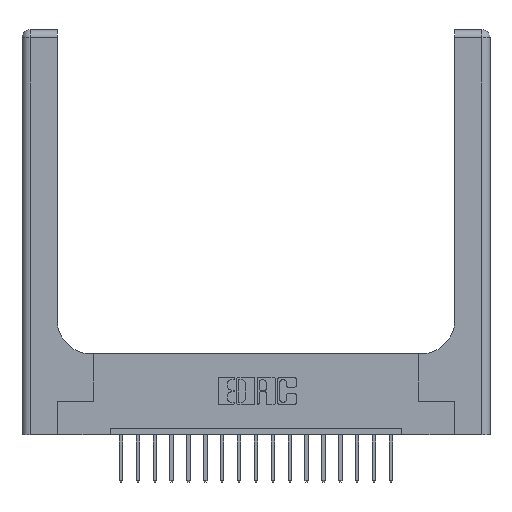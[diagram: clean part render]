
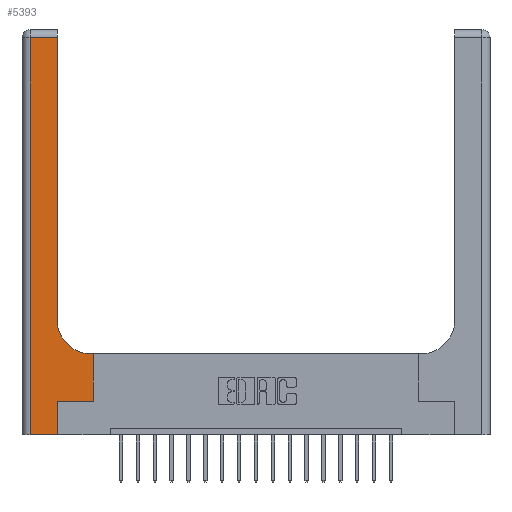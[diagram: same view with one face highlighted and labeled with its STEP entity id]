
A CAD part, top view. The second image highlights one B-rep face of the part: STEP entity #5393.
In plain terms, the highlighted planar face has unit normal (0, 0, 1).
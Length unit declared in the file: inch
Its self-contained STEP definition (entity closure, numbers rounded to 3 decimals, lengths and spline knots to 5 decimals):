
#104 = DIRECTION ( 'NONE',  ( 0., 0., -1. ) ) ;
#293 = FACE_OUTER_BOUND ( 'NONE', #8924, .T. ) ;
#439 = DIRECTION ( 'NONE',  ( 0., 1., 0. ) ) ;
#589 = CARTESIAN_POINT ( 'NONE',  ( 0.26, 0.6, 0.37 ) ) ;
#680 = DIRECTION ( 'NONE',  ( 1., 0., 0. ) ) ;
#683 = ORIENTED_EDGE ( 'NONE', *, *, #4215, .T. ) ;
#714 = DIRECTION ( 'NONE',  ( -1., 0., 0. ) ) ;
#737 = CARTESIAN_POINT ( 'NONE',  ( 0.528, 0.25, 0.37 ) ) ;
#1125 = EDGE_CURVE ( 'NONE', #5862, #8726, #2071, .T. ) ;
#1465 = CARTESIAN_POINT ( 'NONE',  ( 0.528, 0.6, 0.37 ) ) ;
#2071 = LINE ( 'NONE', #589, #18342 ) ;
#2080 = VERTEX_POINT ( 'NONE', #737 ) ;
#2270 = DIRECTION ( 'NONE',  ( -1., 0., 0. ) ) ;
#2566 = CARTESIAN_POINT ( 'NONE',  ( 0.265, 0., 0.37 ) ) ;
#2879 = VERTEX_POINT ( 'NONE', #10970 ) ;
#2986 = ORIENTED_EDGE ( 'NONE', *, *, #13654, .T. ) ;
#3689 = LINE ( 'NONE', #17036, #10026 ) ;
#4020 = DIRECTION ( 'NONE',  ( 1., 0., 0. ) ) ;
#4074 = AXIS2_PLACEMENT_3D ( 'NONE', #7520, #8815, #10492 ) ;
#4215 = EDGE_CURVE ( 'NONE', #8726, #6994, #14821, .T. ) ;
#4394 = VERTEX_POINT ( 'NONE', #2566 ) ;
#4497 = DIRECTION ( 'NONE',  ( 0., 1., 0. ) ) ;
#4581 = VECTOR ( 'NONE', #4020, 39.37008 ) ;
#5181 = CARTESIAN_POINT ( 'NONE',  ( 0.26, 3., 0.37 ) ) ;
#5393 = ADVANCED_FACE ( 'NONE', ( #293 ), #18110, .F. ) ;
#5862 = VERTEX_POINT ( 'NONE', #1465 ) ;
#6149 = DIRECTION ( 'NONE',  ( -1., 0., 0. ) ) ;
#6428 = EDGE_CURVE ( 'NONE', #4394, #15464, #8164, .T. ) ;
#6541 = ORIENTED_EDGE ( 'NONE', *, *, #6428, .T. ) ;
#6583 = CARTESIAN_POINT ( 'NONE',  ( 0.265, 0., 0.37 ) ) ;
#6991 = LINE ( 'NONE', #11636, #4581 ) ;
#6994 = VERTEX_POINT ( 'NONE', #19374 ) ;
#7324 = ORIENTED_EDGE ( 'NONE', *, *, #13899, .T. ) ;
#7430 = LINE ( 'NONE', #13553, #15594 ) ;
#7520 = CARTESIAN_POINT ( 'NONE',  ( 0.51, 0.85, 0.37 ) ) ;
#7566 = CARTESIAN_POINT ( 'NONE',  ( 0.528, 0.25, 0.37 ) ) ;
#7940 = EDGE_CURVE ( 'NONE', #6994, #10862, #8346, .T. ) ;
#8052 = VECTOR ( 'NONE', #680, 39.37008 ) ;
#8164 = LINE ( 'NONE', #6583, #14835 ) ;
#8346 = LINE ( 'NONE', #5181, #12974 ) ;
#8506 = EDGE_CURVE ( 'NONE', #2080, #5862, #12011, .T. ) ;
#8726 = VERTEX_POINT ( 'NONE', #14167 ) ;
#8815 = DIRECTION ( 'NONE',  ( 0., 0., -1. ) ) ;
#8924 = EDGE_LOOP ( 'NONE', ( #10285, #12834, #2986, #18857, #6541, #7324, #13659, #14261, #683 ) ) ;
#10026 = VECTOR ( 'NONE', #714, 39.37008 ) ;
#10285 = ORIENTED_EDGE ( 'NONE', *, *, #7940, .T. ) ;
#10492 = DIRECTION ( 'NONE',  ( 1., 0., 0. ) ) ;
#10862 = VERTEX_POINT ( 'NONE', #15213 ) ;
#10970 = CARTESIAN_POINT ( 'NONE',  ( 0.06, 0., 0.37 ) ) ;
#11636 = CARTESIAN_POINT ( 'NONE',  ( 0., 0., 0.37 ) ) ;
#11687 = AXIS2_PLACEMENT_3D ( 'NONE', #15151, #104, #6149 ) ;
#12011 = LINE ( 'NONE', #7566, #18991 ) ;
#12083 = VERTEX_POINT ( 'NONE', #16537 ) ;
#12834 = ORIENTED_EDGE ( 'NONE', *, *, #18480, .T. ) ;
#12974 = VECTOR ( 'NONE', #17040, 39.37008 ) ;
#13356 = DIRECTION ( 'NONE',  ( 0., -1., 0. ) ) ;
#13553 = CARTESIAN_POINT ( 'NONE',  ( 0.06, 3., 0.37 ) ) ;
#13654 = EDGE_CURVE ( 'NONE', #12083, #2879, #7430, .T. ) ;
#13659 = ORIENTED_EDGE ( 'NONE', *, *, #8506, .T. ) ;
#13899 = EDGE_CURVE ( 'NONE', #15464, #2080, #18690, .T. ) ;
#14167 = CARTESIAN_POINT ( 'NONE',  ( 0.51, 0.6, 0.37 ) ) ;
#14261 = ORIENTED_EDGE ( 'NONE', *, *, #1125, .T. ) ;
#14362 = EDGE_CURVE ( 'NONE', #2879, #4394, #6991, .T. ) ;
#14821 = CIRCLE ( 'NONE', #4074, 0.25 ) ;
#14835 = VECTOR ( 'NONE', #439, 39.37008 ) ;
#15151 = CARTESIAN_POINT ( 'NONE',  ( 0., 3., 0.37 ) ) ;
#15213 = CARTESIAN_POINT ( 'NONE',  ( 0.26, 2.94, 0.37 ) ) ;
#15464 = VERTEX_POINT ( 'NONE', #19103 ) ;
#15594 = VECTOR ( 'NONE', #13356, 39.37008 ) ;
#16537 = CARTESIAN_POINT ( 'NONE',  ( 0.06, 2.94, 0.37 ) ) ;
#17036 = CARTESIAN_POINT ( 'NONE',  ( 0., 2.94, 0.37 ) ) ;
#17040 = DIRECTION ( 'NONE',  ( 0., 1., 0. ) ) ;
#18110 = PLANE ( 'NONE',  #11687 ) ;
#18342 = VECTOR ( 'NONE', #2270, 39.37008 ) ;
#18396 = CARTESIAN_POINT ( 'NONE',  ( 0.265, 0.25, 0.37 ) ) ;
#18480 = EDGE_CURVE ( 'NONE', #10862, #12083, #3689, .T. ) ;
#18690 = LINE ( 'NONE', #18396, #8052 ) ;
#18857 = ORIENTED_EDGE ( 'NONE', *, *, #14362, .T. ) ;
#18991 = VECTOR ( 'NONE', #4497, 39.37008 ) ;
#19103 = CARTESIAN_POINT ( 'NONE',  ( 0.265, 0.25, 0.37 ) ) ;
#19374 = CARTESIAN_POINT ( 'NONE',  ( 0.26, 0.85, 0.37 ) ) ;
